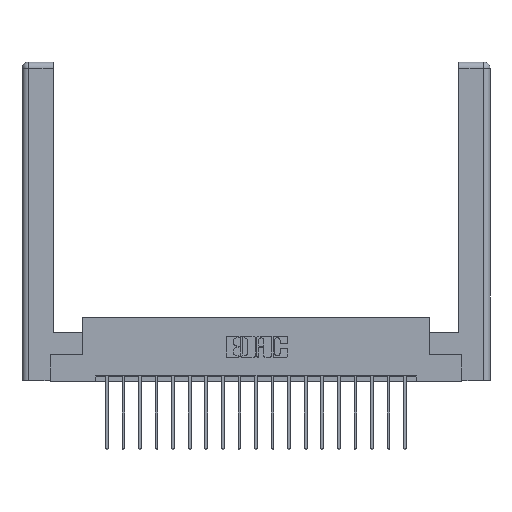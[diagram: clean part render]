
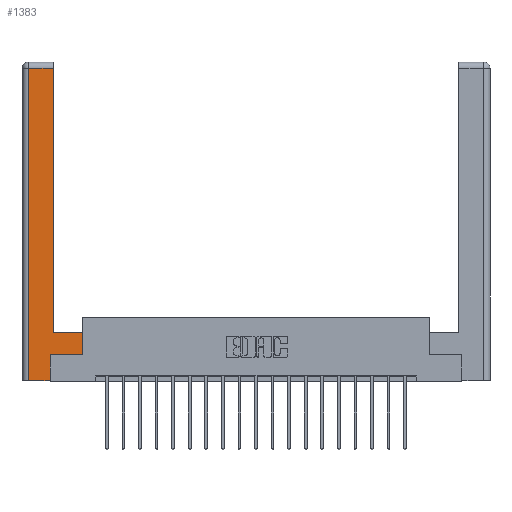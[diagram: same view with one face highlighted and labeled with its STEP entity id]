
A CAD part, top view. The second image highlights one B-rep face of the part: STEP entity #1383.
In plain terms, the highlighted planar face has unit normal (0, 0, 1).
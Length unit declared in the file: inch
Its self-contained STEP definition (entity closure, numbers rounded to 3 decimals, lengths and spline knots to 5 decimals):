
#88 = VERTEX_POINT ( 'NONE', #5517 ) ;
#1383 = ADVANCED_FACE ( 'NONE', ( #1537 ), #11823, .F. ) ;
#1385 = DIRECTION ( 'NONE',  ( -1., 0., 0. ) ) ;
#1537 = FACE_OUTER_BOUND ( 'NONE', #10761, .T. ) ;
#2428 = DIRECTION ( 'NONE',  ( 0., 1., 0. ) ) ;
#2447 = DIRECTION ( 'NONE',  ( 0., 1., 0. ) ) ;
#2961 = CARTESIAN_POINT ( 'NONE',  ( 0.565, 0.245, 0. ) ) ;
#3567 = ORIENTED_EDGE ( 'NONE', *, *, #19881, .T. ) ;
#3735 = EDGE_CURVE ( 'NONE', #16819, #88, #20165, .T. ) ;
#3841 = CARTESIAN_POINT ( 'NONE',  ( 0.295, 3., 0. ) ) ;
#4146 = EDGE_CURVE ( 'NONE', #6548, #16819, #11747, .T. ) ;
#4240 = ORIENTED_EDGE ( 'NONE', *, *, #14258, .T. ) ;
#4281 = DIRECTION ( 'NONE',  ( 1., 0., 0. ) ) ;
#4406 = EDGE_CURVE ( 'NONE', #18142, #13945, #10013, .T. ) ;
#4466 = ORIENTED_EDGE ( 'NONE', *, *, #4406, .T. ) ;
#4555 = CARTESIAN_POINT ( 'NONE',  ( 0.565, 0.245, 0. ) ) ;
#4747 = ORIENTED_EDGE ( 'NONE', *, *, #4146, .T. ) ;
#4769 = DIRECTION ( 'NONE',  ( -1., 0., 0. ) ) ;
#5266 = EDGE_CURVE ( 'NONE', #13945, #13782, #18687, .T. ) ;
#5517 = CARTESIAN_POINT ( 'NONE',  ( 0.295, 2.94, 0. ) ) ;
#5645 = CARTESIAN_POINT ( 'NONE',  ( 0., 0., 0. ) ) ;
#5851 = LINE ( 'NONE', #10660, #18918 ) ;
#6118 = DIRECTION ( 'NONE',  ( 0., 1., 0. ) ) ;
#6215 = EDGE_CURVE ( 'NONE', #9136, #9594, #19866, .T. ) ;
#6548 = VERTEX_POINT ( 'NONE', #19527 ) ;
#6591 = CARTESIAN_POINT ( 'NONE',  ( 0.0615, 2.94, 0. ) ) ;
#6842 = CARTESIAN_POINT ( 'NONE',  ( 0.265, 0., 0. ) ) ;
#6859 = VECTOR ( 'NONE', #1385, 39.37008 ) ;
#7106 = VECTOR ( 'NONE', #11967, 39.37008 ) ;
#7115 = ORIENTED_EDGE ( 'NONE', *, *, #5266, .T. ) ;
#7279 = AXIS2_PLACEMENT_3D ( 'NONE', #5645, #17963, #18102 ) ;
#8019 = LINE ( 'NONE', #12468, #11935 ) ;
#8662 = CARTESIAN_POINT ( 'NONE',  ( 0.295, 0.45, 0. ) ) ;
#9136 = VERTEX_POINT ( 'NONE', #15366 ) ;
#9594 = VERTEX_POINT ( 'NONE', #4555 ) ;
#10013 = LINE ( 'NONE', #11172, #10764 ) ;
#10660 = CARTESIAN_POINT ( 'NONE',  ( 0.565, 0.45, 0. ) ) ;
#10761 = EDGE_LOOP ( 'NONE', ( #19107, #3567, #4466, #7115, #4240, #12342, #15115, #4747 ) ) ;
#10764 = VECTOR ( 'NONE', #15787, 39.37008 ) ;
#11172 = CARTESIAN_POINT ( 'NONE',  ( 0.0615, 0., 0. ) ) ;
#11441 = VECTOR ( 'NONE', #4281, 39.37008 ) ;
#11747 = LINE ( 'NONE', #16653, #6859 ) ;
#11823 = PLANE ( 'NONE',  #7279 ) ;
#11935 = VECTOR ( 'NONE', #4769, 39.37008 ) ;
#11967 = DIRECTION ( 'NONE',  ( 1., 0., 0. ) ) ;
#12342 = ORIENTED_EDGE ( 'NONE', *, *, #6215, .T. ) ;
#12468 = CARTESIAN_POINT ( 'NONE',  ( 0.0615, 2.94, 0. ) ) ;
#13749 = VECTOR ( 'NONE', #2428, 39.37008 ) ;
#13782 = VERTEX_POINT ( 'NONE', #6842 ) ;
#13945 = VERTEX_POINT ( 'NONE', #18791 ) ;
#14258 = EDGE_CURVE ( 'NONE', #13782, #9136, #17952, .T. ) ;
#15115 = ORIENTED_EDGE ( 'NONE', *, *, #19073, .T. ) ;
#15366 = CARTESIAN_POINT ( 'NONE',  ( 0.265, 0.245, 0. ) ) ;
#15787 = DIRECTION ( 'NONE',  ( 0., -1., 0. ) ) ;
#16476 = VECTOR ( 'NONE', #2447, 39.37008 ) ;
#16653 = CARTESIAN_POINT ( 'NONE',  ( 0.295, 0.45, 0. ) ) ;
#16819 = VERTEX_POINT ( 'NONE', #8662 ) ;
#17952 = LINE ( 'NONE', #19804, #16476 ) ;
#17963 = DIRECTION ( 'NONE',  ( 0., 0., -1. ) ) ;
#18102 = DIRECTION ( 'NONE',  ( -1., 0., 0. ) ) ;
#18142 = VERTEX_POINT ( 'NONE', #6591 ) ;
#18390 = CARTESIAN_POINT ( 'NONE',  ( 0.265, 0., 0. ) ) ;
#18687 = LINE ( 'NONE', #18390, #7106 ) ;
#18791 = CARTESIAN_POINT ( 'NONE',  ( 0.0615, 0., 0. ) ) ;
#18918 = VECTOR ( 'NONE', #6118, 39.37008 ) ;
#19073 = EDGE_CURVE ( 'NONE', #9594, #6548, #5851, .T. ) ;
#19107 = ORIENTED_EDGE ( 'NONE', *, *, #3735, .T. ) ;
#19527 = CARTESIAN_POINT ( 'NONE',  ( 0.565, 0.45, 0. ) ) ;
#19804 = CARTESIAN_POINT ( 'NONE',  ( 0.265, 0.245, 0. ) ) ;
#19866 = LINE ( 'NONE', #2961, #11441 ) ;
#19881 = EDGE_CURVE ( 'NONE', #88, #18142, #8019, .T. ) ;
#20165 = LINE ( 'NONE', #3841, #13749 ) ;
